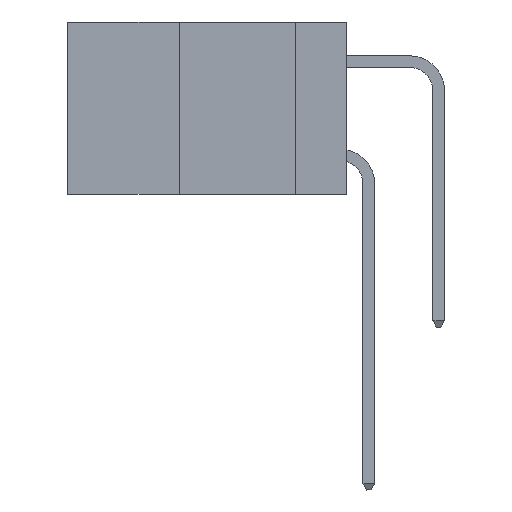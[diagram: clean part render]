
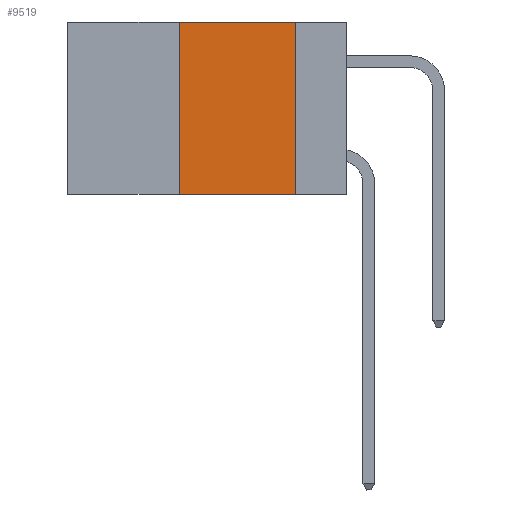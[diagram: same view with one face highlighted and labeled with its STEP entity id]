
A CAD part, left-side view. The second image highlights one B-rep face of the part: STEP entity #9519.
In plain terms, the highlighted planar face has unit normal (-1, 0, 0).
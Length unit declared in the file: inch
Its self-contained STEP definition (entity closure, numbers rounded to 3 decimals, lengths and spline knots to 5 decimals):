
#1551 = VERTEX_POINT ( 'NONE', #40036 ) ;
#5640 = AXIS2_PLACEMENT_3D ( 'NONE', #33103, #13474, #9328 ) ;
#7155 = ORIENTED_EDGE ( 'NONE', *, *, #8500, .F. ) ;
#7250 = VERTEX_POINT ( 'NONE', #17134 ) ;
#8247 = LINE ( 'NONE', #19705, #15850 ) ;
#8500 = EDGE_CURVE ( 'NONE', #7250, #1551, #15400, .T. ) ;
#8546 = ORIENTED_EDGE ( 'NONE', *, *, #44637, .F. ) ;
#9017 = DIRECTION ( 'NONE',  ( 0., 0., -1. ) ) ;
#9328 = DIRECTION ( 'NONE',  ( 0., 0., -1. ) ) ;
#9519 = ADVANCED_FACE ( 'NONE', ( #23490 ), #40281, .F. ) ;
#10400 = EDGE_CURVE ( 'NONE', #16028, #7250, #8247, .T. ) ;
#13474 = DIRECTION ( 'NONE',  ( 1., 0., 0. ) ) ;
#15400 = LINE ( 'NONE', #26336, #39375 ) ;
#15850 = VECTOR ( 'NONE', #30458, 39.37008 ) ;
#16028 = VERTEX_POINT ( 'NONE', #27047 ) ;
#16255 = VECTOR ( 'NONE', #42441, 39.37008 ) ;
#16986 = EDGE_CURVE ( 'NONE', #23950, #1551, #38667, .T. ) ;
#17134 = CARTESIAN_POINT ( 'NONE',  ( 0., 0.11, 0. ) ) ;
#19705 = CARTESIAN_POINT ( 'NONE',  ( 0., 0.6, 0. ) ) ;
#20202 = VECTOR ( 'NONE', #25966, 39.37008 ) ;
#22244 = LINE ( 'NONE', #42288, #16255 ) ;
#23293 = ORIENTED_EDGE ( 'NONE', *, *, #10400, .F. ) ;
#23490 = FACE_OUTER_BOUND ( 'NONE', #35989, .T. ) ;
#23950 = VERTEX_POINT ( 'NONE', #36727 ) ;
#25495 = CARTESIAN_POINT ( 'NONE',  ( 0., 0.6, -0.37 ) ) ;
#25966 = DIRECTION ( 'NONE',  ( 0., -1., 0. ) ) ;
#26336 = CARTESIAN_POINT ( 'NONE',  ( 0., 0.11, 0. ) ) ;
#27047 = CARTESIAN_POINT ( 'NONE',  ( 0., 0.36, 0. ) ) ;
#30458 = DIRECTION ( 'NONE',  ( 0., -1., 0. ) ) ;
#33103 = CARTESIAN_POINT ( 'NONE',  ( 0., 0.6, 0. ) ) ;
#35989 = EDGE_LOOP ( 'NONE', ( #7155, #23293, #8546, #43476 ) ) ;
#36727 = CARTESIAN_POINT ( 'NONE',  ( 0., 0.36, -0.37 ) ) ;
#38667 = LINE ( 'NONE', #25495, #20202 ) ;
#39375 = VECTOR ( 'NONE', #9017, 39.37008 ) ;
#40036 = CARTESIAN_POINT ( 'NONE',  ( 0., 0.11, -0.37 ) ) ;
#40281 = PLANE ( 'NONE',  #5640 ) ;
#42288 = CARTESIAN_POINT ( 'NONE',  ( 0., 0.36, 0. ) ) ;
#42441 = DIRECTION ( 'NONE',  ( 0., 0., 1. ) ) ;
#43476 = ORIENTED_EDGE ( 'NONE', *, *, #16986, .T. ) ;
#44637 = EDGE_CURVE ( 'NONE', #23950, #16028, #22244, .T. ) ;
